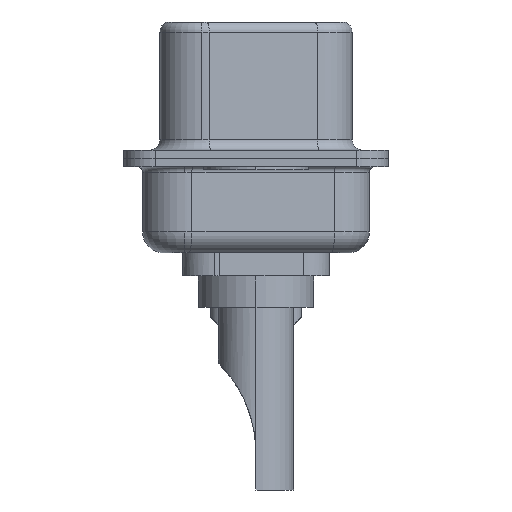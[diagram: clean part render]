
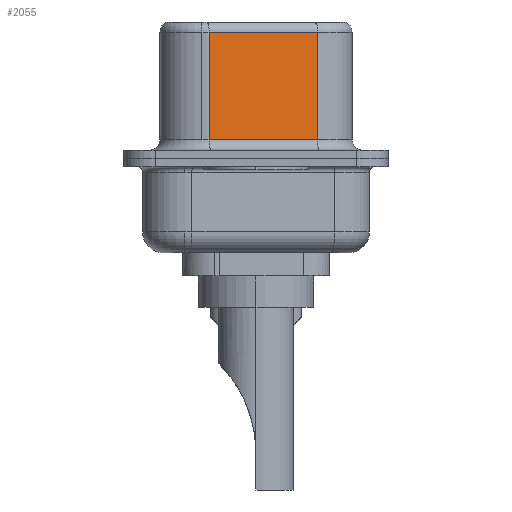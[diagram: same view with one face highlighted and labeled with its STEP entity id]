
A CAD part, left-side view. The second image highlights one B-rep face of the part: STEP entity #2055.
In plain terms, the highlighted planar face has unit normal (-0.985, -0.174, 0).
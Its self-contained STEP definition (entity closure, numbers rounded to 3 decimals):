
#917 = LINE ( 'NONE', #6850, #10892 ) ;
#1604 = ORIENTED_EDGE ( 'NONE', *, *, #9043, .F. ) ;
#2055 = ADVANCED_FACE ( 'NONE', ( #8124 ), #7132, .F. ) ;
#2400 = VERTEX_POINT ( 'NONE', #13927 ) ;
#2771 = LINE ( 'NONE', #5496, #11948 ) ;
#3859 = LINE ( 'NONE', #5042, #9424 ) ;
#3888 = VECTOR ( 'NONE', #5545, 1000. ) ;
#5042 = CARTESIAN_POINT ( 'NONE',  ( 3.675, 2.233, 6.52 ) ) ;
#5496 = CARTESIAN_POINT ( 'NONE',  ( 4.585, -2.927, 6.02 ) ) ;
#5545 = DIRECTION ( 'NONE',  ( 0.174, -0.985, 0. ) ) ;
#5968 = ORIENTED_EDGE ( 'NONE', *, *, #13867, .T. ) ;
#6035 = AXIS2_PLACEMENT_3D ( 'NONE', #7366, #12698, #6854 ) ;
#6850 = CARTESIAN_POINT ( 'NONE',  ( 4.585, -2.927, 6.52 ) ) ;
#6854 = DIRECTION ( 'NONE',  ( -0.174, 0.985, 0. ) ) ;
#6947 = EDGE_CURVE ( 'NONE', #2400, #7299, #2771, .T. ) ;
#7132 = PLANE ( 'NONE',  #6035 ) ;
#7299 = VERTEX_POINT ( 'NONE', #10246 ) ;
#7366 = CARTESIAN_POINT ( 'NONE',  ( 4.585, -2.927, 6.52 ) ) ;
#7397 = EDGE_CURVE ( 'NONE', #11090, #7474, #13402, .T. ) ;
#7474 = VERTEX_POINT ( 'NONE', #10769 ) ;
#8124 = FACE_OUTER_BOUND ( 'NONE', #11559, .T. ) ;
#8232 = CARTESIAN_POINT ( 'NONE',  ( 3.675, 2.233, 0.9 ) ) ;
#8902 = DIRECTION ( 'NONE',  ( -0.174, 0.985, 0. ) ) ;
#9043 = EDGE_CURVE ( 'NONE', #2400, #7474, #917, .T. ) ;
#9125 = ORIENTED_EDGE ( 'NONE', *, *, #7397, .T. ) ;
#9259 = DIRECTION ( 'NONE',  ( 0., 0., -1. ) ) ;
#9424 = VECTOR ( 'NONE', #13400, 1000. ) ;
#10246 = CARTESIAN_POINT ( 'NONE',  ( 3.675, 2.233, 6.02 ) ) ;
#10769 = CARTESIAN_POINT ( 'NONE',  ( 4.585, -2.927, 0.9 ) ) ;
#10892 = VECTOR ( 'NONE', #9259, 1000. ) ;
#11090 = VERTEX_POINT ( 'NONE', #8232 ) ;
#11559 = EDGE_LOOP ( 'NONE', ( #1604, #11585, #5968, #9125 ) ) ;
#11562 = CARTESIAN_POINT ( 'NONE',  ( 4.585, -2.927, 0.9 ) ) ;
#11585 = ORIENTED_EDGE ( 'NONE', *, *, #6947, .T. ) ;
#11948 = VECTOR ( 'NONE', #8902, 1000. ) ;
#12698 = DIRECTION ( 'NONE',  ( 0.985, 0.174, 0. ) ) ;
#13400 = DIRECTION ( 'NONE',  ( 0., 0., -1. ) ) ;
#13402 = LINE ( 'NONE', #11562, #3888 ) ;
#13867 = EDGE_CURVE ( 'NONE', #7299, #11090, #3859, .T. ) ;
#13927 = CARTESIAN_POINT ( 'NONE',  ( 4.585, -2.927, 6.02 ) ) ;
